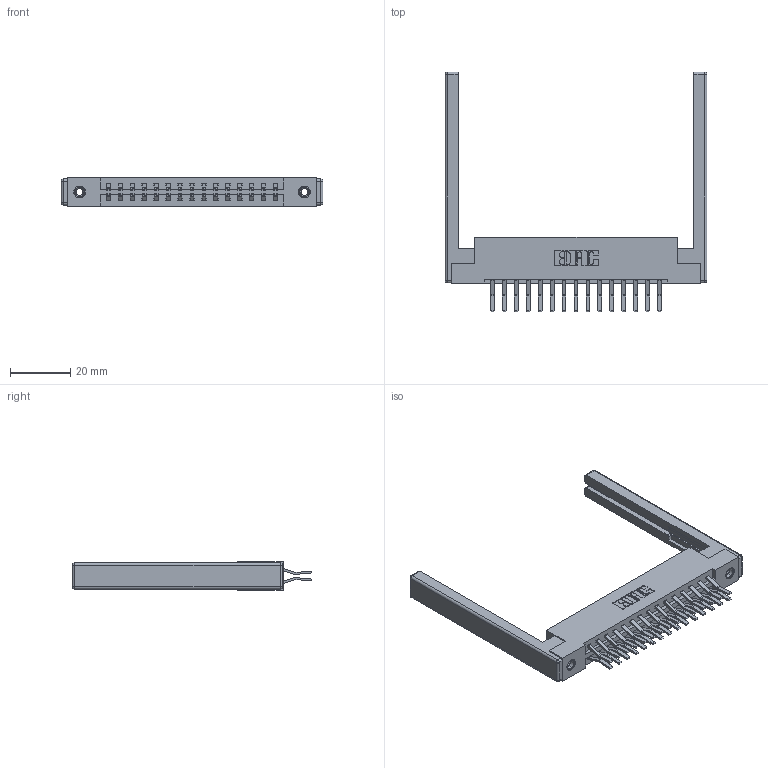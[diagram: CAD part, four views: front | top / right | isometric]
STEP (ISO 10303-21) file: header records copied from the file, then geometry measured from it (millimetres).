
FILE_DESCRIPTION (( 'STEP AP203' ), '1' );
FILE_NAME ('387-030-560-268.STEP', '2019-10-17T15:15:30', ( '' ), ( '' ), 'SwSTEP 2.0', 'SolidWorks 2016', '' );
FILE_SCHEMA (( 'CONFIG_CONTROL_DESIGN' ));
Length unit declared in the file: inch
Products named in the file (5): 307-220-068; 387-030-560-268; 337 Part_Flush Mounting Lugs - 0.156 Dia-TI; 345-292-001_560 Tail; 345-250-001_345-250-001-102
Assembly tree (35 placements, depth 2):
  387-030-560-268
    337 Part_Flush Mounting Lugs - 0.156 Dia-TI
    345-292-001_560 Tail  x30
    345-250-001_345-250-001-102  x2
    307-220-068  x2
Bounding box: 86.87 x 79.52 x 9.4 mm (x, y, z)
Volume: 13376.9 mm3; surface area: 14506.8 mm2
Topology: 35 solids, 35 shells, 1948 faces, 5711 edges, 3746 vertices
Faces by surface type: plane 1298, cylinder 626, cone 12, sphere 8, torus 4
Entity records: 17970 total; most frequent: CARTESIAN_POINT 3015, ORIENTED_EDGE 2940, DIRECTION 2688, EDGE_CURVE 1470, LINE 1288, VECTOR 1288, VERTEX_POINT 970, AXIS2_PLACEMENT_3D 700
